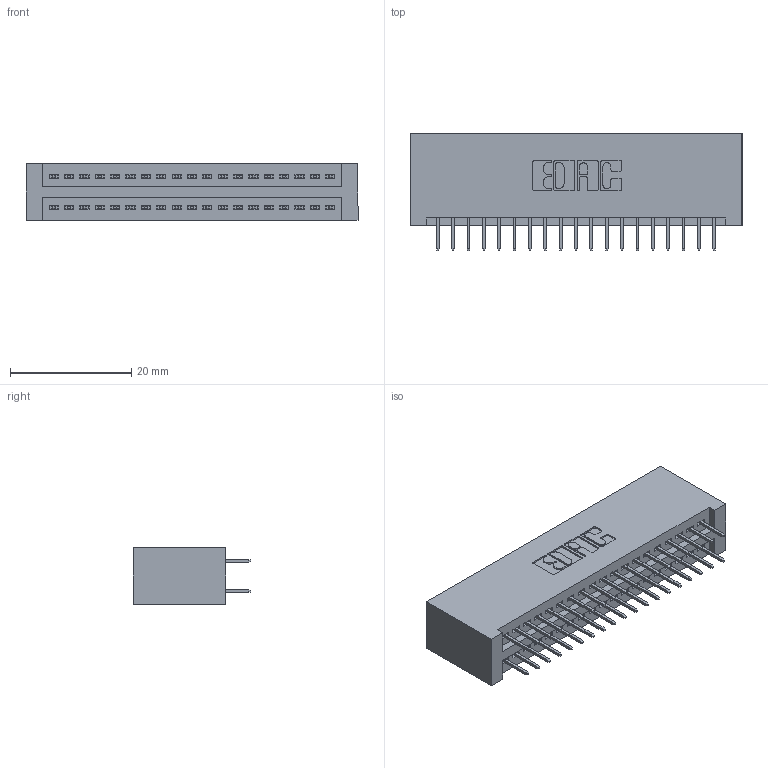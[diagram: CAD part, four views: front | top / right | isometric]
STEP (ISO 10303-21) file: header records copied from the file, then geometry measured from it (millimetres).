
FILE_DESCRIPTION (( 'STEP AP203' ), '1' );
FILE_NAME ('395-038-524-201.STEP', '2018-11-14T02:45:20', ( '' ), ( '' ), 'SwSTEP 2.0', 'SolidWorks 2016', '' );
FILE_SCHEMA (( 'CONFIG_CONTROL_DESIGN' ));
Length unit declared in the file: inch
Products named in the file (3): 345-292-001_345-293-124; 395-038-524-201; 345 Part_No Mounting Lugs
Assembly tree (39 placements, depth 2):
  395-038-524-201
    345 Part_No Mounting Lugs
    345-292-001_345-293-124  x38
Bounding box: 54.86 x 19.35 x 9.4 mm (x, y, z)
Volume: 5674.5 mm3; surface area: 8093.8 mm2
Topology: 39 solids, 39 shells, 2170 faces, 6131 edges, 3934 vertices
Faces by surface type: plane 1558, cylinder 612
Entity records: 17801 total; most frequent: CARTESIAN_POINT 3004, ORIENTED_EDGE 2938, DIRECTION 2673, EDGE_CURVE 1469, VECTOR 1273, LINE 1273, VERTEX_POINT 974, AXIS2_PLACEMENT_3D 700
